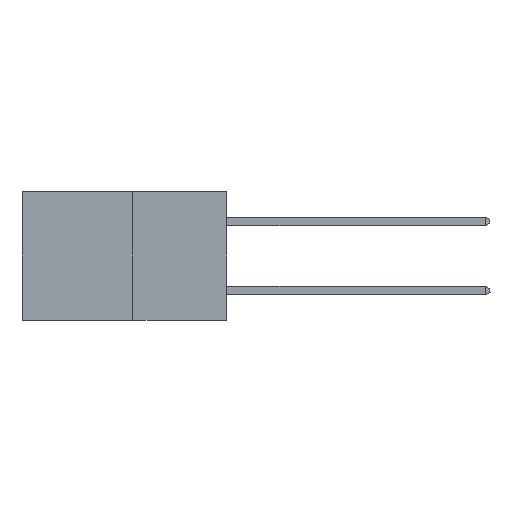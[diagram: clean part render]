
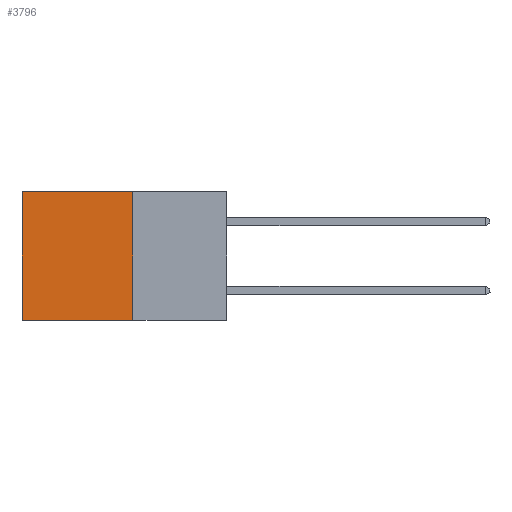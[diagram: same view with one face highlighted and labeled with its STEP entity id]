
A CAD part, left-side view. The second image highlights one B-rep face of the part: STEP entity #3796.
In plain terms, the highlighted planar face has unit normal (-1, 0, 0).
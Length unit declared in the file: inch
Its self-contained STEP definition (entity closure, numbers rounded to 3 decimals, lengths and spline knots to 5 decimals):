
#176 = EDGE_CURVE ( 'NONE', #10008, #391, #10244, .T. ) ;
#204 = AXIS2_PLACEMENT_3D ( 'NONE', #6517, #1741, #7247 ) ;
#391 = VERTEX_POINT ( 'NONE', #1019 ) ;
#557 = VERTEX_POINT ( 'NONE', #8185 ) ;
#728 = DIRECTION ( 'NONE',  ( 0., 0., -1. ) ) ;
#744 = LINE ( 'NONE', #9923, #924 ) ;
#785 = PLANE ( 'NONE',  #204 ) ;
#924 = VECTOR ( 'NONE', #7128, 39.37008 ) ;
#1019 = CARTESIAN_POINT ( 'NONE',  ( 0.277, 0.27, -0.37 ) ) ;
#1245 = ORIENTED_EDGE ( 'NONE', *, *, #176, .F. ) ;
#1253 = EDGE_CURVE ( 'NONE', #391, #557, #744, .T. ) ;
#1741 = DIRECTION ( 'NONE',  ( 1., 0., 0. ) ) ;
#1872 = EDGE_CURVE ( 'NONE', #9907, #557, #8304, .T. ) ;
#2856 = DIRECTION ( 'NONE',  ( 0., 1., 0. ) ) ;
#3562 = ORIENTED_EDGE ( 'NONE', *, *, #1253, .F. ) ;
#3647 = CARTESIAN_POINT ( 'NONE',  ( 0.277, 0.27, 0. ) ) ;
#3703 = ORIENTED_EDGE ( 'NONE', *, *, #1872, .T. ) ;
#3796 = ADVANCED_FACE ( 'NONE', ( #5885 ), #785, .F. ) ;
#3996 = CARTESIAN_POINT ( 'NONE',  ( 0.277, 0.59, -0.37 ) ) ;
#5885 = FACE_OUTER_BOUND ( 'NONE', #7172, .T. ) ;
#6222 = CARTESIAN_POINT ( 'NONE',  ( 0.277, 0.27, 0. ) ) ;
#6246 = VECTOR ( 'NONE', #2856, 39.37008 ) ;
#6289 = DIRECTION ( 'NONE',  ( 0., 0., -1. ) ) ;
#6517 = CARTESIAN_POINT ( 'NONE',  ( 0.277, 0.27, -0.37 ) ) ;
#6856 = CARTESIAN_POINT ( 'NONE',  ( 0.277, 0.59, 0. ) ) ;
#7128 = DIRECTION ( 'NONE',  ( 0., 1., 0. ) ) ;
#7172 = EDGE_LOOP ( 'NONE', ( #3703, #3562, #1245, #7355 ) ) ;
#7247 = DIRECTION ( 'NONE',  ( 0., 0., -1. ) ) ;
#7355 = ORIENTED_EDGE ( 'NONE', *, *, #8767, .T. ) ;
#8040 = VECTOR ( 'NONE', #6289, 39.37008 ) ;
#8185 = CARTESIAN_POINT ( 'NONE',  ( 0.277, 0.59, -0.37 ) ) ;
#8304 = LINE ( 'NONE', #3996, #10289 ) ;
#8388 = LINE ( 'NONE', #3647, #6246 ) ;
#8767 = EDGE_CURVE ( 'NONE', #10008, #9907, #8388, .T. ) ;
#9316 = CARTESIAN_POINT ( 'NONE',  ( 0.277, 0.27, -0.37 ) ) ;
#9907 = VERTEX_POINT ( 'NONE', #6856 ) ;
#9923 = CARTESIAN_POINT ( 'NONE',  ( 0.277, 0.27, -0.37 ) ) ;
#10008 = VERTEX_POINT ( 'NONE', #6222 ) ;
#10244 = LINE ( 'NONE', #9316, #8040 ) ;
#10289 = VECTOR ( 'NONE', #728, 39.37008 ) ;
